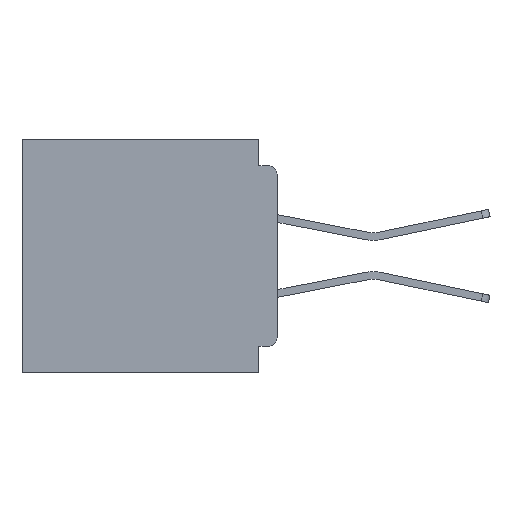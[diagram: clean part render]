
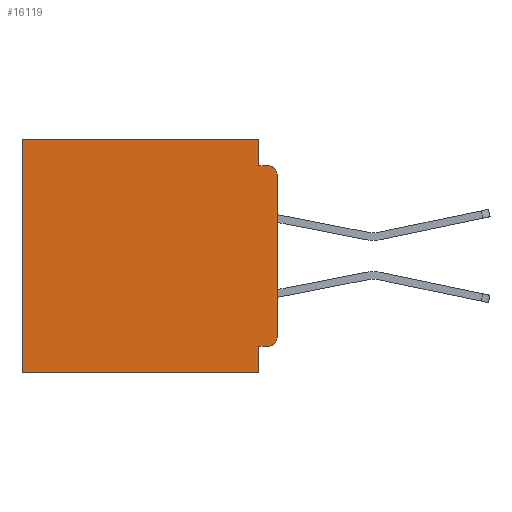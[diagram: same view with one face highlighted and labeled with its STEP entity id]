
A CAD part, left-side view. The second image highlights one B-rep face of the part: STEP entity #16119.
In plain terms, the highlighted planar face has unit normal (-1, 0, 0).
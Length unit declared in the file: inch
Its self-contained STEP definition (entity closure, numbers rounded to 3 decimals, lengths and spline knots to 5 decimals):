
#139 = CARTESIAN_POINT ( 'NONE',  ( 0.3, 0., -0.4 ) ) ;
#211 = CARTESIAN_POINT ( 'NONE',  ( 0.3, 0., -0.4 ) ) ;
#325 = VECTOR ( 'NONE', #20186, 39.37008 ) ;
#451 = VERTEX_POINT ( 'NONE', #24373 ) ;
#460 = ORIENTED_EDGE ( 'NONE', *, *, #12668, .T. ) ;
#506 = ORIENTED_EDGE ( 'NONE', *, *, #20954, .F. ) ;
#1398 = CARTESIAN_POINT ( 'NONE',  ( 0.3, 0.031, -0.045 ) ) ;
#2311 = VERTEX_POINT ( 'NONE', #9723 ) ;
#2665 = CARTESIAN_POINT ( 'NONE',  ( 0.3, 0., -0.06 ) ) ;
#2912 = CIRCLE ( 'NONE', #34210, 0.015 ) ;
#3108 = EDGE_CURVE ( 'NONE', #451, #26008, #38968, .T. ) ;
#3489 = DIRECTION ( 'NONE',  ( 0., 0., -1. ) ) ;
#3927 = LINE ( 'NONE', #27539, #22207 ) ;
#4874 = VECTOR ( 'NONE', #19872, 39.37008 ) ;
#5498 = DIRECTION ( 'NONE',  ( -1., 0., 0. ) ) ;
#5876 = LINE ( 'NONE', #19729, #4874 ) ;
#6670 = VERTEX_POINT ( 'NONE', #2665 ) ;
#8986 = ORIENTED_EDGE ( 'NONE', *, *, #25152, .T. ) ;
#8989 = LINE ( 'NONE', #38656, #33830 ) ;
#9411 = VECTOR ( 'NONE', #19571, 39.37008 ) ;
#9723 = CARTESIAN_POINT ( 'NONE',  ( 0.3, 0.031, 0. ) ) ;
#11178 = ORIENTED_EDGE ( 'NONE', *, *, #37349, .T. ) ;
#12075 = VECTOR ( 'NONE', #23827, 39.37008 ) ;
#12169 = VECTOR ( 'NONE', #37597, 39.37008 ) ;
#12668 = EDGE_CURVE ( 'NONE', #39438, #26008, #8989, .T. ) ;
#12798 = EDGE_CURVE ( 'NONE', #18797, #451, #5876, .T. ) ;
#13436 = EDGE_LOOP ( 'NONE', ( #506, #16211, #37087, #32644, #11178, #460, #28688, #36321, #27229, #8986 ) ) ;
#14027 = AXIS2_PLACEMENT_3D ( 'NONE', #14163, #36930, #17410 ) ;
#14031 = CARTESIAN_POINT ( 'NONE',  ( 0.3, 0., -0.045 ) ) ;
#14163 = CARTESIAN_POINT ( 'NONE',  ( 0.3, 0.015, -0.34 ) ) ;
#14846 = AXIS2_PLACEMENT_3D ( 'NONE', #211, #22915, #3489 ) ;
#16119 = ADVANCED_FACE ( 'NONE', ( #34134 ), #29321, .F. ) ;
#16211 = ORIENTED_EDGE ( 'NONE', *, *, #39172, .T. ) ;
#16575 = LINE ( 'NONE', #36425, #325 ) ;
#16954 = CARTESIAN_POINT ( 'NONE',  ( 0.3, 0.015, -0.355 ) ) ;
#17410 = DIRECTION ( 'NONE',  ( 0., 0., -1. ) ) ;
#18797 = VERTEX_POINT ( 'NONE', #33817 ) ;
#18984 = LINE ( 'NONE', #139, #9411 ) ;
#19571 = DIRECTION ( 'NONE',  ( 0., 0., -1. ) ) ;
#19729 = CARTESIAN_POINT ( 'NONE',  ( 0.3, 0.031, -0.4 ) ) ;
#19872 = DIRECTION ( 'NONE',  ( 0., 0., -1. ) ) ;
#20186 = DIRECTION ( 'NONE',  ( 0., 1., 0. ) ) ;
#20954 = EDGE_CURVE ( 'NONE', #6670, #37742, #18984, .T. ) ;
#22207 = VECTOR ( 'NONE', #40428, 39.37008 ) ;
#22915 = DIRECTION ( 'NONE',  ( 1., 0., 0. ) ) ;
#23031 = CARTESIAN_POINT ( 'NONE',  ( 0.3, 0.437, 0. ) ) ;
#23136 = VERTEX_POINT ( 'NONE', #1398 ) ;
#23827 = DIRECTION ( 'NONE',  ( 0., -1., 0. ) ) ;
#24245 = CIRCLE ( 'NONE', #14027, 0.015 ) ;
#24373 = CARTESIAN_POINT ( 'NONE',  ( 0.3, 0.031, -0.4 ) ) ;
#24929 = CARTESIAN_POINT ( 'NONE',  ( 0.3, 0.015, -0.06 ) ) ;
#25119 = EDGE_CURVE ( 'NONE', #23136, #36858, #41508, .T. ) ;
#25152 = EDGE_CURVE ( 'NONE', #27536, #37742, #24245, .T. ) ;
#25231 = EDGE_CURVE ( 'NONE', #2311, #23136, #3927, .T. ) ;
#26008 = VERTEX_POINT ( 'NONE', #32036 ) ;
#26228 = EDGE_CURVE ( 'NONE', #27536, #18797, #16575, .T. ) ;
#27229 = ORIENTED_EDGE ( 'NONE', *, *, #26228, .F. ) ;
#27536 = VERTEX_POINT ( 'NONE', #16954 ) ;
#27539 = CARTESIAN_POINT ( 'NONE',  ( 0.3, 0.031, 0. ) ) ;
#28203 = DIRECTION ( 'NONE',  ( 0., 0., -1. ) ) ;
#28310 = DIRECTION ( 'NONE',  ( 0., 1., 0. ) ) ;
#28688 = ORIENTED_EDGE ( 'NONE', *, *, #3108, .F. ) ;
#29321 = PLANE ( 'NONE',  #14846 ) ;
#31373 = VECTOR ( 'NONE', #28310, 39.37008 ) ;
#32036 = CARTESIAN_POINT ( 'NONE',  ( 0.3, 0.437, -0.4 ) ) ;
#32644 = ORIENTED_EDGE ( 'NONE', *, *, #25231, .F. ) ;
#33817 = CARTESIAN_POINT ( 'NONE',  ( 0.3, 0.031, -0.355 ) ) ;
#33830 = VECTOR ( 'NONE', #41873, 39.37008 ) ;
#34134 = FACE_OUTER_BOUND ( 'NONE', #13436, .T. ) ;
#34210 = AXIS2_PLACEMENT_3D ( 'NONE', #24929, #5498, #28203 ) ;
#34303 = CARTESIAN_POINT ( 'NONE',  ( 0.3, 0., 0. ) ) ;
#36321 = ORIENTED_EDGE ( 'NONE', *, *, #12798, .F. ) ;
#36425 = CARTESIAN_POINT ( 'NONE',  ( 0.3, 0., -0.355 ) ) ;
#36858 = VERTEX_POINT ( 'NONE', #41560 ) ;
#36867 = CARTESIAN_POINT ( 'NONE',  ( 0.3, 0., -0.34 ) ) ;
#36930 = DIRECTION ( 'NONE',  ( -1., 0., 0. ) ) ;
#37087 = ORIENTED_EDGE ( 'NONE', *, *, #25119, .F. ) ;
#37101 = LINE ( 'NONE', #34303, #12169 ) ;
#37349 = EDGE_CURVE ( 'NONE', #2311, #39438, #37101, .T. ) ;
#37597 = DIRECTION ( 'NONE',  ( 0., 1., 0. ) ) ;
#37742 = VERTEX_POINT ( 'NONE', #36867 ) ;
#38175 = CARTESIAN_POINT ( 'NONE',  ( 0.3, 0., -0.4 ) ) ;
#38656 = CARTESIAN_POINT ( 'NONE',  ( 0.3, 0.437, -0.4 ) ) ;
#38968 = LINE ( 'NONE', #38175, #31373 ) ;
#39172 = EDGE_CURVE ( 'NONE', #6670, #36858, #2912, .T. ) ;
#39438 = VERTEX_POINT ( 'NONE', #23031 ) ;
#40428 = DIRECTION ( 'NONE',  ( 0., 0., -1. ) ) ;
#41508 = LINE ( 'NONE', #14031, #12075 ) ;
#41560 = CARTESIAN_POINT ( 'NONE',  ( 0.3, 0.015, -0.045 ) ) ;
#41873 = DIRECTION ( 'NONE',  ( 0., 0., -1. ) ) ;
